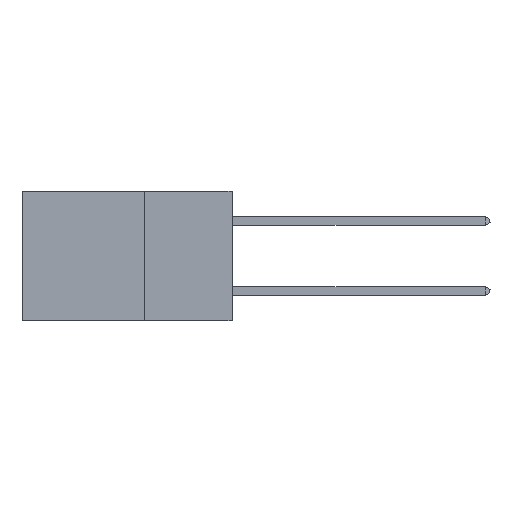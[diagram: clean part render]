
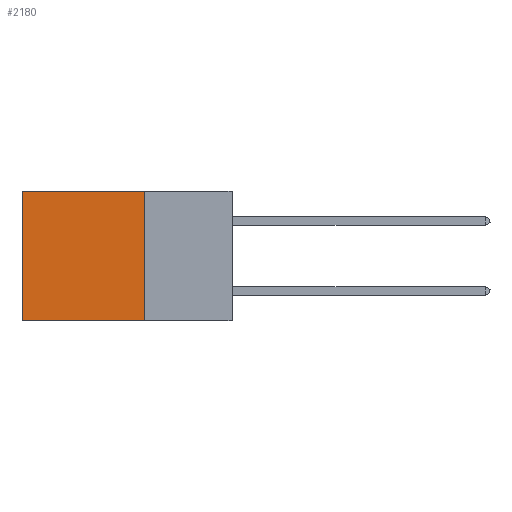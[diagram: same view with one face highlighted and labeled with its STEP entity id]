
A CAD part, left-side view. The second image highlights one B-rep face of the part: STEP entity #2180.
In plain terms, the highlighted planar face has unit normal (-1, 0, 0).
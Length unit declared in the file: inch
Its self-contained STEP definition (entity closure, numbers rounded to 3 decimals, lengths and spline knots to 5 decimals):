
#1668 = LINE ( 'NONE', #29753, #31833 ) ;
#2180 = ADVANCED_FACE ( 'NONE', ( #12343 ), #5728, .F. ) ;
#2883 = ORIENTED_EDGE ( 'NONE', *, *, #16977, .T. ) ;
#3032 = DIRECTION ( 'NONE',  ( 0., 1., 0. ) ) ;
#4869 = VECTOR ( 'NONE', #16492, 39.37008 ) ;
#5346 = AXIS2_PLACEMENT_3D ( 'NONE', #10964, #25893, #10642 ) ;
#5728 = PLANE ( 'NONE',  #5346 ) ;
#6821 = VERTEX_POINT ( 'NONE', #20741 ) ;
#8852 = EDGE_CURVE ( 'NONE', #6821, #10508, #9855, .T. ) ;
#9855 = LINE ( 'NONE', #23264, #14813 ) ;
#10508 = VERTEX_POINT ( 'NONE', #29274 ) ;
#10642 = DIRECTION ( 'NONE',  ( 0., 0., -1. ) ) ;
#10920 = CARTESIAN_POINT ( 'NONE',  ( 0.2875, 0.25, 0. ) ) ;
#10964 = CARTESIAN_POINT ( 'NONE',  ( 0.2875, 0.25, 0. ) ) ;
#11708 = VECTOR ( 'NONE', #23591, 39.37008 ) ;
#11867 = CARTESIAN_POINT ( 'NONE',  ( 0.2875, 0.25, 0. ) ) ;
#12343 = FACE_OUTER_BOUND ( 'NONE', #12705, .T. ) ;
#12705 = EDGE_LOOP ( 'NONE', ( #14531, #31451, #15821, #2883 ) ) ;
#13389 = DIRECTION ( 'NONE',  ( 0., 0., -1. ) ) ;
#13834 = EDGE_CURVE ( 'NONE', #23473, #19926, #31479, .T. ) ;
#14531 = ORIENTED_EDGE ( 'NONE', *, *, #8852, .T. ) ;
#14813 = VECTOR ( 'NONE', #13389, 39.37008 ) ;
#14987 = EDGE_CURVE ( 'NONE', #19926, #10508, #1668, .T. ) ;
#15821 = ORIENTED_EDGE ( 'NONE', *, *, #13834, .F. ) ;
#16492 = DIRECTION ( 'NONE',  ( 0., 1., 0. ) ) ;
#16977 = EDGE_CURVE ( 'NONE', #23473, #6821, #29584, .T. ) ;
#19926 = VERTEX_POINT ( 'NONE', #26849 ) ;
#20741 = CARTESIAN_POINT ( 'NONE',  ( 0.2875, 0.6, 0. ) ) ;
#21726 = CARTESIAN_POINT ( 'NONE',  ( 0.2875, 0.25, 0. ) ) ;
#23264 = CARTESIAN_POINT ( 'NONE',  ( 0.2875, 0.6, 0. ) ) ;
#23473 = VERTEX_POINT ( 'NONE', #11867 ) ;
#23591 = DIRECTION ( 'NONE',  ( 0., 0., -1. ) ) ;
#25893 = DIRECTION ( 'NONE',  ( 1., 0., 0. ) ) ;
#26849 = CARTESIAN_POINT ( 'NONE',  ( 0.2875, 0.25, -0.37 ) ) ;
#29274 = CARTESIAN_POINT ( 'NONE',  ( 0.2875, 0.6, -0.37 ) ) ;
#29584 = LINE ( 'NONE', #21726, #4869 ) ;
#29753 = CARTESIAN_POINT ( 'NONE',  ( 0.2875, 0.25, -0.37 ) ) ;
#31451 = ORIENTED_EDGE ( 'NONE', *, *, #14987, .F. ) ;
#31479 = LINE ( 'NONE', #10920, #11708 ) ;
#31833 = VECTOR ( 'NONE', #3032, 39.37008 ) ;
